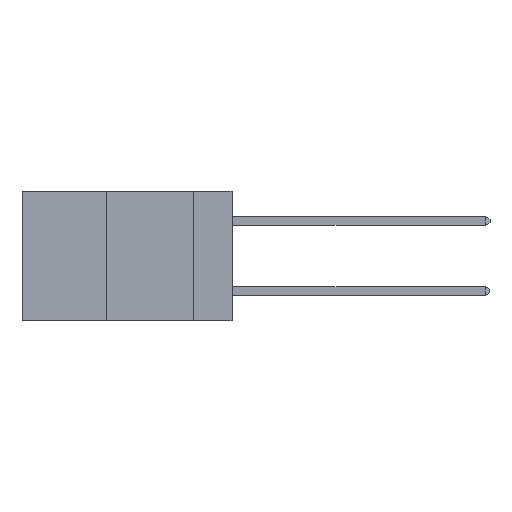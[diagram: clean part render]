
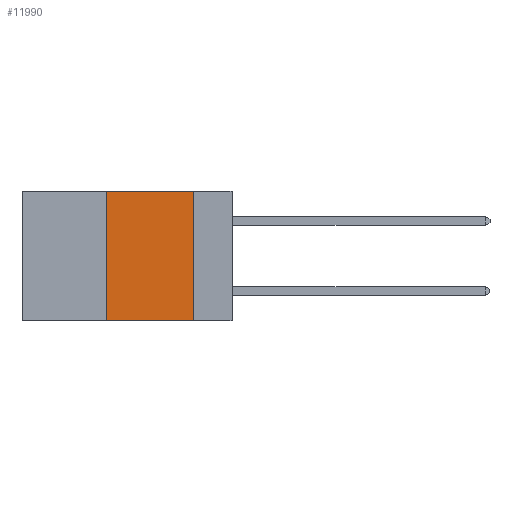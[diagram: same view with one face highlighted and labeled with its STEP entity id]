
A CAD part, left-side view. The second image highlights one B-rep face of the part: STEP entity #11990.
In plain terms, the highlighted planar face has unit normal (-1, 0, 0).
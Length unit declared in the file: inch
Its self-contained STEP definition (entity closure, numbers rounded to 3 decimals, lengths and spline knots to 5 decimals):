
#49 = VERTEX_POINT ( 'NONE', #5730 ) ;
#145 = CARTESIAN_POINT ( 'NONE',  ( 0., 0.6, 0. ) ) ;
#721 = CARTESIAN_POINT ( 'NONE',  ( 0., 0.6, 0. ) ) ;
#975 = EDGE_LOOP ( 'NONE', ( #11591, #6720, #11902, #4478 ) ) ;
#1062 = CARTESIAN_POINT ( 'NONE',  ( 0., 0.11, -0.37 ) ) ;
#1100 = LINE ( 'NONE', #721, #6028 ) ;
#1155 = DIRECTION ( 'NONE',  ( 0., 0., -1. ) ) ;
#1560 = DIRECTION ( 'NONE',  ( 0., 0., 1. ) ) ;
#1784 = EDGE_CURVE ( 'NONE', #49, #11966, #2309, .T. ) ;
#1823 = VECTOR ( 'NONE', #1560, 39.37008 ) ;
#1906 = VERTEX_POINT ( 'NONE', #10330 ) ;
#2309 = LINE ( 'NONE', #4828, #6884 ) ;
#2441 = EDGE_CURVE ( 'NONE', #49, #5884, #4463, .T. ) ;
#3774 = EDGE_CURVE ( 'NONE', #1906, #11966, #10347, .T. ) ;
#3820 = CARTESIAN_POINT ( 'NONE',  ( 0., 0.36, 0. ) ) ;
#3863 = EDGE_CURVE ( 'NONE', #5884, #1906, #1100, .T. ) ;
#4198 = FACE_OUTER_BOUND ( 'NONE', #975, .T. ) ;
#4463 = LINE ( 'NONE', #11658, #1823 ) ;
#4478 = ORIENTED_EDGE ( 'NONE', *, *, #1784, .T. ) ;
#4828 = CARTESIAN_POINT ( 'NONE',  ( 0., 0.6, -0.37 ) ) ;
#5730 = CARTESIAN_POINT ( 'NONE',  ( 0., 0.36, -0.37 ) ) ;
#5884 = VERTEX_POINT ( 'NONE', #3820 ) ;
#6028 = VECTOR ( 'NONE', #12407, 39.37008 ) ;
#6064 = PLANE ( 'NONE',  #8967 ) ;
#6720 = ORIENTED_EDGE ( 'NONE', *, *, #3863, .F. ) ;
#6884 = VECTOR ( 'NONE', #9815, 39.37008 ) ;
#6980 = DIRECTION ( 'NONE',  ( 1., 0., 0. ) ) ;
#7383 = CARTESIAN_POINT ( 'NONE',  ( 0., 0.11, 0. ) ) ;
#7712 = VECTOR ( 'NONE', #10351, 39.37008 ) ;
#8967 = AXIS2_PLACEMENT_3D ( 'NONE', #145, #6980, #1155 ) ;
#9815 = DIRECTION ( 'NONE',  ( 0., -1., 0. ) ) ;
#10330 = CARTESIAN_POINT ( 'NONE',  ( 0., 0.11, 0. ) ) ;
#10347 = LINE ( 'NONE', #7383, #7712 ) ;
#10351 = DIRECTION ( 'NONE',  ( 0., 0., -1. ) ) ;
#11591 = ORIENTED_EDGE ( 'NONE', *, *, #3774, .F. ) ;
#11658 = CARTESIAN_POINT ( 'NONE',  ( 0., 0.36, 0. ) ) ;
#11902 = ORIENTED_EDGE ( 'NONE', *, *, #2441, .F. ) ;
#11966 = VERTEX_POINT ( 'NONE', #1062 ) ;
#11990 = ADVANCED_FACE ( 'NONE', ( #4198 ), #6064, .F. ) ;
#12407 = DIRECTION ( 'NONE',  ( 0., -1., 0. ) ) ;
